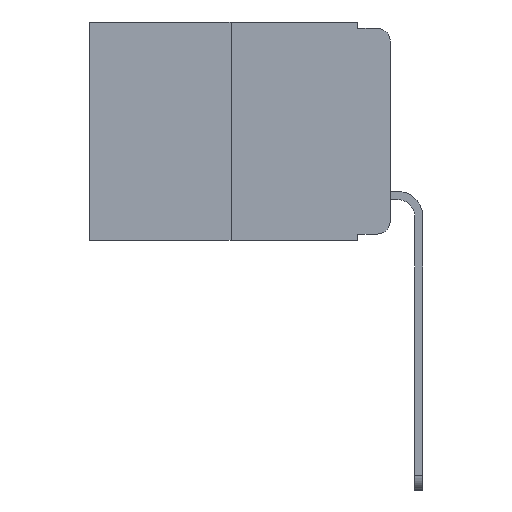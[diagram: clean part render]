
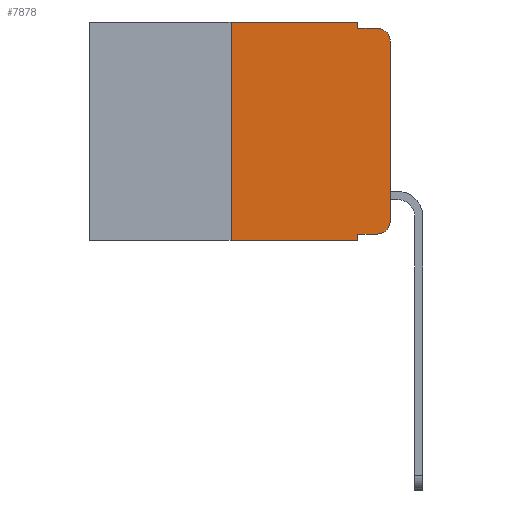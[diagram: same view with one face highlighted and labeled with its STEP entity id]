
A CAD part, left-side view. The second image highlights one B-rep face of the part: STEP entity #7878.
In plain terms, the highlighted planar face has unit normal (-1, 0, 0).
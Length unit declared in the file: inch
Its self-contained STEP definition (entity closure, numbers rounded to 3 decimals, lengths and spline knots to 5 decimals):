
#21 = EDGE_CURVE ( 'NONE', #12571, #2929, #6525, .T. ) ;
#40 = VECTOR ( 'NONE', #12283, 39.37008 ) ;
#78 = LINE ( 'NONE', #4428, #7780 ) ;
#84 = ORIENTED_EDGE ( 'NONE', *, *, #6706, .T. ) ;
#114 = DIRECTION ( 'NONE',  ( 0., 0., -1. ) ) ;
#148 = ORIENTED_EDGE ( 'NONE', *, *, #12663, .F. ) ;
#503 = VERTEX_POINT ( 'NONE', #8731 ) ;
#619 = DIRECTION ( 'NONE',  ( -1., 0., 0. ) ) ;
#945 = EDGE_CURVE ( 'NONE', #11540, #8651, #1889, .T. ) ;
#962 = VECTOR ( 'NONE', #2927, 39.37008 ) ;
#978 = CARTESIAN_POINT ( 'NONE',  ( 0., 0., -0.313 ) ) ;
#1552 = EDGE_CURVE ( 'NONE', #1580, #10488, #2668, .T. ) ;
#1580 = VERTEX_POINT ( 'NONE', #3513 ) ;
#1852 = ORIENTED_EDGE ( 'NONE', *, *, #1552, .F. ) ;
#1889 = LINE ( 'NONE', #5365, #12645 ) ;
#1961 = ORIENTED_EDGE ( 'NONE', *, *, #11026, .F. ) ;
#2117 = CARTESIAN_POINT ( 'NONE',  ( 0., 0.473, -0.343 ) ) ;
#2320 = CARTESIAN_POINT ( 'NONE',  ( 0., 0.25, -0.343 ) ) ;
#2325 = ORIENTED_EDGE ( 'NONE', *, *, #945, .T. ) ;
#2668 = LINE ( 'NONE', #3473, #13455 ) ;
#2745 = CARTESIAN_POINT ( 'NONE',  ( 0., 0.051, -0.333 ) ) ;
#2927 = DIRECTION ( 'NONE',  ( 0., -1., 0. ) ) ;
#2929 = VERTEX_POINT ( 'NONE', #3808 ) ;
#3038 = AXIS2_PLACEMENT_3D ( 'NONE', #9459, #5284, #12567 ) ;
#3274 = VECTOR ( 'NONE', #6268, 39.37008 ) ;
#3473 = CARTESIAN_POINT ( 'NONE',  ( 0., 0.473, 0. ) ) ;
#3513 = CARTESIAN_POINT ( 'NONE',  ( 0., 0.25, 0. ) ) ;
#3590 = LINE ( 'NONE', #5215, #3274 ) ;
#3808 = CARTESIAN_POINT ( 'NONE',  ( 0., 0.051, -0.343 ) ) ;
#3904 = AXIS2_PLACEMENT_3D ( 'NONE', #12605, #6372, #114 ) ;
#4413 = ORIENTED_EDGE ( 'NONE', *, *, #10916, .T. ) ;
#4428 = CARTESIAN_POINT ( 'NONE',  ( 0., 0., 0. ) ) ;
#4755 = DIRECTION ( 'NONE',  ( 0., -1., 0. ) ) ;
#5017 = CARTESIAN_POINT ( 'NONE',  ( 0., 0.051, 0. ) ) ;
#5124 = CIRCLE ( 'NONE', #13261, 0.02 ) ;
#5215 = CARTESIAN_POINT ( 'NONE',  ( 0., 0.25, 0. ) ) ;
#5222 = VECTOR ( 'NONE', #9243, 39.37008 ) ;
#5276 = LINE ( 'NONE', #5017, #40 ) ;
#5284 = DIRECTION ( 'NONE',  ( 1., 0., 0. ) ) ;
#5365 = CARTESIAN_POINT ( 'NONE',  ( 0., 0.051, -0.333 ) ) ;
#5935 = EDGE_CURVE ( 'NONE', #503, #9247, #12664, .T. ) ;
#6268 = DIRECTION ( 'NONE',  ( 0., 0., 1. ) ) ;
#6372 = DIRECTION ( 'NONE',  ( -1., 0., 0. ) ) ;
#6525 = LINE ( 'NONE', #2117, #962 ) ;
#6535 = DIRECTION ( 'NONE',  ( 0., 0., 1. ) ) ;
#6632 = DIRECTION ( 'NONE',  ( 0., -1., 0. ) ) ;
#6706 = EDGE_CURVE ( 'NONE', #13060, #503, #78, .T. ) ;
#6884 = CARTESIAN_POINT ( 'NONE',  ( 0., 0.02, -0.313 ) ) ;
#7216 = VECTOR ( 'NONE', #8723, 39.37008 ) ;
#7414 = LINE ( 'NONE', #8180, #5222 ) ;
#7612 = FACE_OUTER_BOUND ( 'NONE', #12674, .T. ) ;
#7672 = CARTESIAN_POINT ( 'NONE',  ( 0., 0.051, -0.01 ) ) ;
#7734 = CARTESIAN_POINT ( 'NONE',  ( 0., 0.02, -0.01 ) ) ;
#7780 = VECTOR ( 'NONE', #6535, 39.37008 ) ;
#7878 = ADVANCED_FACE ( 'NONE', ( #7612 ), #11511, .F. ) ;
#7936 = DIRECTION ( 'NONE',  ( 0., 0., -1. ) ) ;
#8180 = CARTESIAN_POINT ( 'NONE',  ( 0., 0.051, 0. ) ) ;
#8651 = VERTEX_POINT ( 'NONE', #8846 ) ;
#8723 = DIRECTION ( 'NONE',  ( 0., -1., 0. ) ) ;
#8731 = CARTESIAN_POINT ( 'NONE',  ( 0., 0., -0.03 ) ) ;
#8846 = CARTESIAN_POINT ( 'NONE',  ( 0., 0.02, -0.333 ) ) ;
#9243 = DIRECTION ( 'NONE',  ( 0., 0., -1. ) ) ;
#9247 = VERTEX_POINT ( 'NONE', #7734 ) ;
#9459 = CARTESIAN_POINT ( 'NONE',  ( 0., 0.473, 0. ) ) ;
#9468 = VERTEX_POINT ( 'NONE', #13205 ) ;
#9762 = ORIENTED_EDGE ( 'NONE', *, *, #5935, .T. ) ;
#9993 = LINE ( 'NONE', #7672, #7216 ) ;
#10004 = ORIENTED_EDGE ( 'NONE', *, *, #13280, .F. ) ;
#10488 = VERTEX_POINT ( 'NONE', #11403 ) ;
#10916 = EDGE_CURVE ( 'NONE', #8651, #13060, #5124, .T. ) ;
#11026 = EDGE_CURVE ( 'NONE', #11540, #2929, #5276, .T. ) ;
#11403 = CARTESIAN_POINT ( 'NONE',  ( 0., 0.051, 0. ) ) ;
#11511 = PLANE ( 'NONE',  #3038 ) ;
#11540 = VERTEX_POINT ( 'NONE', #2745 ) ;
#11797 = EDGE_CURVE ( 'NONE', #12571, #1580, #3590, .T. ) ;
#12024 = ORIENTED_EDGE ( 'NONE', *, *, #21, .T. ) ;
#12283 = DIRECTION ( 'NONE',  ( 0., 0., -1. ) ) ;
#12567 = DIRECTION ( 'NONE',  ( 0., 0., -1. ) ) ;
#12571 = VERTEX_POINT ( 'NONE', #2320 ) ;
#12605 = CARTESIAN_POINT ( 'NONE',  ( 0., 0.02, -0.03 ) ) ;
#12645 = VECTOR ( 'NONE', #4755, 39.37008 ) ;
#12663 = EDGE_CURVE ( 'NONE', #9468, #9247, #9993, .T. ) ;
#12664 = CIRCLE ( 'NONE', #3904, 0.02 ) ;
#12674 = EDGE_LOOP ( 'NONE', ( #84, #9762, #148, #10004, #1852, #12782, #12024, #1961, #2325, #4413 ) ) ;
#12782 = ORIENTED_EDGE ( 'NONE', *, *, #11797, .F. ) ;
#13060 = VERTEX_POINT ( 'NONE', #978 ) ;
#13205 = CARTESIAN_POINT ( 'NONE',  ( 0., 0.051, -0.01 ) ) ;
#13261 = AXIS2_PLACEMENT_3D ( 'NONE', #6884, #619, #7936 ) ;
#13280 = EDGE_CURVE ( 'NONE', #10488, #9468, #7414, .T. ) ;
#13455 = VECTOR ( 'NONE', #6632, 39.37008 ) ;
